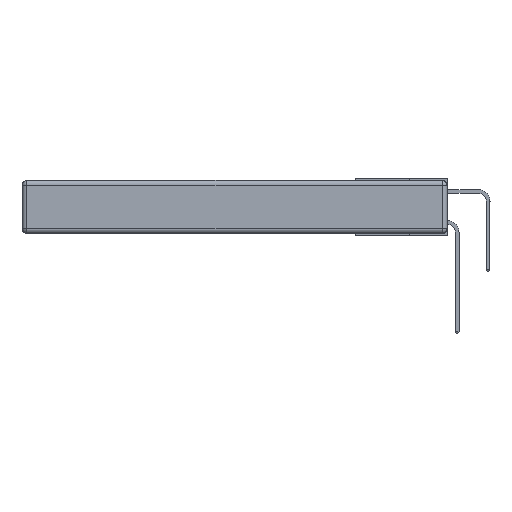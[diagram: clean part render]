
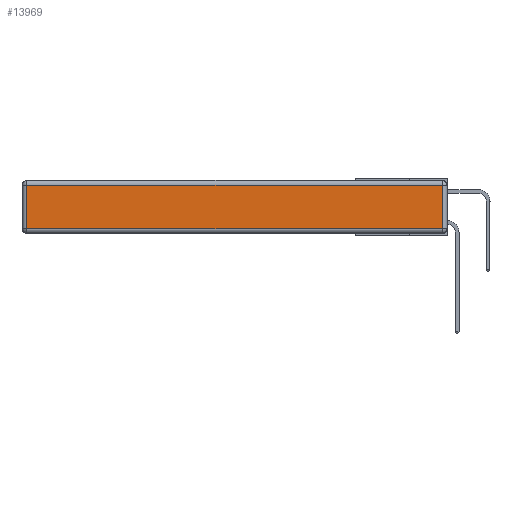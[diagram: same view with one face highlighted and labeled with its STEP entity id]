
A CAD part, left-side view. The second image highlights one B-rep face of the part: STEP entity #13969.
In plain terms, the highlighted planar face has unit normal (-1, 0, 0).
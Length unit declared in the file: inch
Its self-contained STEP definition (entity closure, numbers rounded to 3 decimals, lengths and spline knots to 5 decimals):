
#417 = CARTESIAN_POINT ( 'NONE',  ( 0., 2.72, -0.03 ) ) ;
#597 = PLANE ( 'NONE',  #5074 ) ;
#670 = FACE_OUTER_BOUND ( 'NONE', #5729, .T. ) ;
#767 = CARTESIAN_POINT ( 'NONE',  ( 0., 0., -0.313 ) ) ;
#2736 = DIRECTION ( 'NONE',  ( 0., 0., 1. ) ) ;
#2741 = DIRECTION ( 'NONE',  ( 0., -1., 0. ) ) ;
#3396 = ORIENTED_EDGE ( 'NONE', *, *, #11871, .T. ) ;
#5074 = AXIS2_PLACEMENT_3D ( 'NONE', #10171, #16216, #2736 ) ;
#5151 = VECTOR ( 'NONE', #20468, 39.37008 ) ;
#5729 = EDGE_LOOP ( 'NONE', ( #17713, #10783, #3396, #6615 ) ) ;
#6152 = CARTESIAN_POINT ( 'NONE',  ( 0., 0.03, -0.343 ) ) ;
#6491 = EDGE_CURVE ( 'NONE', #17090, #24711, #23755, .T. ) ;
#6615 = ORIENTED_EDGE ( 'NONE', *, *, #19042, .T. ) ;
#8228 = LINE ( 'NONE', #8572, #5151 ) ;
#8572 = CARTESIAN_POINT ( 'NONE',  ( 0., 2.75, -0.03 ) ) ;
#9756 = EDGE_CURVE ( 'NONE', #22373, #17090, #16344, .T. ) ;
#10171 = CARTESIAN_POINT ( 'NONE',  ( 0., 0., -0.343 ) ) ;
#10783 = ORIENTED_EDGE ( 'NONE', *, *, #6491, .T. ) ;
#10823 = DIRECTION ( 'NONE',  ( 0., 0., -1. ) ) ;
#11847 = VERTEX_POINT ( 'NONE', #417 ) ;
#11871 = EDGE_CURVE ( 'NONE', #24711, #11847, #8228, .T. ) ;
#13969 = ADVANCED_FACE ( 'NONE', ( #670 ), #597, .T. ) ;
#15401 = VECTOR ( 'NONE', #2741, 39.37008 ) ;
#16216 = DIRECTION ( 'NONE',  ( -1., 0., 0. ) ) ;
#16344 = LINE ( 'NONE', #767, #15401 ) ;
#17090 = VERTEX_POINT ( 'NONE', #18702 ) ;
#17427 = CARTESIAN_POINT ( 'NONE',  ( 0., 0.03, -0.03 ) ) ;
#17691 = LINE ( 'NONE', #18899, #19888 ) ;
#17713 = ORIENTED_EDGE ( 'NONE', *, *, #9756, .T. ) ;
#18228 = CARTESIAN_POINT ( 'NONE',  ( 0., 2.72, -0.313 ) ) ;
#18702 = CARTESIAN_POINT ( 'NONE',  ( 0., 0.03, -0.313 ) ) ;
#18899 = CARTESIAN_POINT ( 'NONE',  ( 0., 2.72, -0.343 ) ) ;
#19042 = EDGE_CURVE ( 'NONE', #11847, #22373, #17691, .T. ) ;
#19888 = VECTOR ( 'NONE', #10823, 39.37008 ) ;
#19930 = DIRECTION ( 'NONE',  ( 0., 0., 1. ) ) ;
#20468 = DIRECTION ( 'NONE',  ( 0., 1., 0. ) ) ;
#21625 = VECTOR ( 'NONE', #19930, 39.37008 ) ;
#22373 = VERTEX_POINT ( 'NONE', #18228 ) ;
#23755 = LINE ( 'NONE', #6152, #21625 ) ;
#24711 = VERTEX_POINT ( 'NONE', #17427 ) ;
